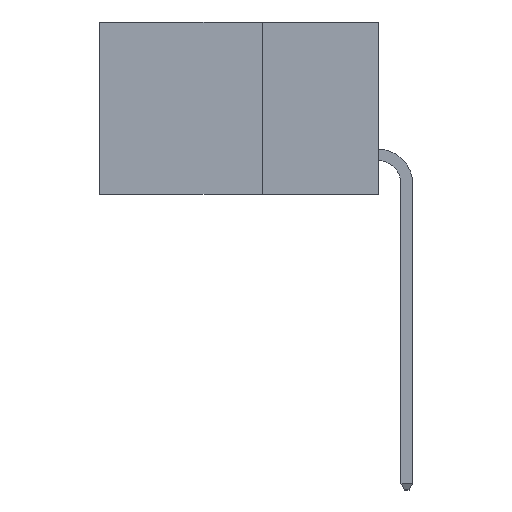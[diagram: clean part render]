
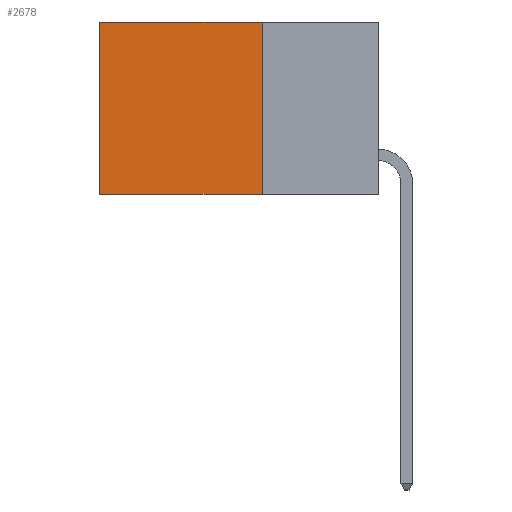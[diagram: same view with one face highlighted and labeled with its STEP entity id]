
A CAD part, left-side view. The second image highlights one B-rep face of the part: STEP entity #2678.
In plain terms, the highlighted planar face has unit normal (-1, 0, 0).
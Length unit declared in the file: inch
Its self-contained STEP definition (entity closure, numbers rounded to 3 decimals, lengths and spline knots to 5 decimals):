
#655 = EDGE_CURVE ( 'NONE', #2065, #10549, #4084, .T. ) ;
#1151 = EDGE_CURVE ( 'NONE', #7525, #2048, #10731, .T. ) ;
#1287 = VECTOR ( 'NONE', #9769, 39.37008 ) ;
#1414 = VECTOR ( 'NONE', #11133, 39.37008 ) ;
#2048 = VERTEX_POINT ( 'NONE', #2758 ) ;
#2065 = VERTEX_POINT ( 'NONE', #3551 ) ;
#2462 = DIRECTION ( 'NONE',  ( 0., 0., -1. ) ) ;
#2678 = ADVANCED_FACE ( 'NONE', ( #11093 ), #10112, .F. ) ;
#2758 = CARTESIAN_POINT ( 'NONE',  ( 0.2615, 0.6, -0.37 ) ) ;
#3551 = CARTESIAN_POINT ( 'NONE',  ( 0.2615, 0.25, 0. ) ) ;
#4084 = LINE ( 'NONE', #10790, #1414 ) ;
#5494 = ORIENTED_EDGE ( 'NONE', *, *, #8548, .T. ) ;
#6031 = CARTESIAN_POINT ( 'NONE',  ( 0.2615, 0.6, 0. ) ) ;
#6050 = DIRECTION ( 'NONE',  ( 0., 1., 0. ) ) ;
#6535 = EDGE_CURVE ( 'NONE', #2065, #7525, #11333, .T. ) ;
#7090 = EDGE_LOOP ( 'NONE', ( #5494, #7950, #10321, #8237 ) ) ;
#7525 = VERTEX_POINT ( 'NONE', #11781 ) ;
#7950 = ORIENTED_EDGE ( 'NONE', *, *, #1151, .F. ) ;
#8175 = CARTESIAN_POINT ( 'NONE',  ( 0.2615, 0.25, -0.37 ) ) ;
#8237 = ORIENTED_EDGE ( 'NONE', *, *, #655, .T. ) ;
#8548 = EDGE_CURVE ( 'NONE', #10549, #2048, #8948, .T. ) ;
#8909 = CARTESIAN_POINT ( 'NONE',  ( 0.2615, 0.6, -0.37 ) ) ;
#8948 = LINE ( 'NONE', #8909, #1287 ) ;
#9769 = DIRECTION ( 'NONE',  ( 0., 0., -1. ) ) ;
#9987 = DIRECTION ( 'NONE',  ( 0., 0., -1. ) ) ;
#10033 = DIRECTION ( 'NONE',  ( 1., 0., 0. ) ) ;
#10112 = PLANE ( 'NONE',  #11118 ) ;
#10321 = ORIENTED_EDGE ( 'NONE', *, *, #6535, .F. ) ;
#10420 = CARTESIAN_POINT ( 'NONE',  ( 0.2615, 0.25, -0.37 ) ) ;
#10436 = VECTOR ( 'NONE', #6050, 39.37008 ) ;
#10549 = VERTEX_POINT ( 'NONE', #6031 ) ;
#10731 = LINE ( 'NONE', #11593, #10436 ) ;
#10790 = CARTESIAN_POINT ( 'NONE',  ( 0.2615, 0.25, 0. ) ) ;
#11093 = FACE_OUTER_BOUND ( 'NONE', #7090, .T. ) ;
#11118 = AXIS2_PLACEMENT_3D ( 'NONE', #10420, #10033, #9987 ) ;
#11133 = DIRECTION ( 'NONE',  ( 0., 1., 0. ) ) ;
#11333 = LINE ( 'NONE', #8175, #11607 ) ;
#11593 = CARTESIAN_POINT ( 'NONE',  ( 0.2615, 0.25, -0.37 ) ) ;
#11607 = VECTOR ( 'NONE', #2462, 39.37008 ) ;
#11781 = CARTESIAN_POINT ( 'NONE',  ( 0.2615, 0.25, -0.37 ) ) ;
